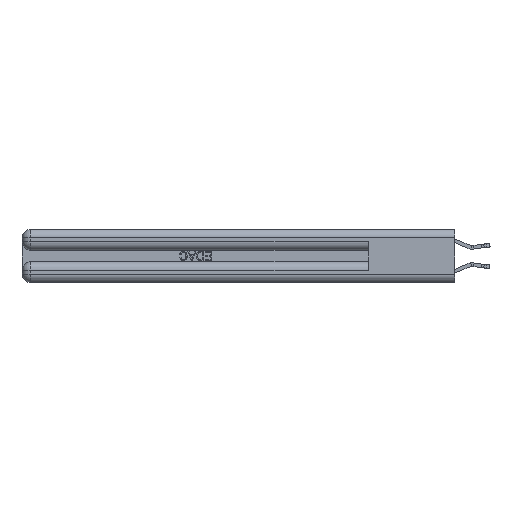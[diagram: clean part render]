
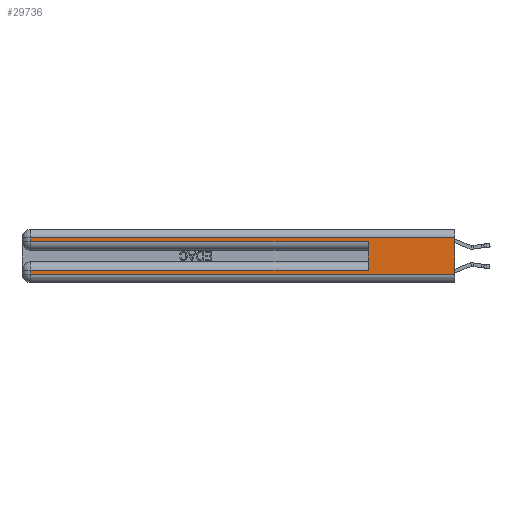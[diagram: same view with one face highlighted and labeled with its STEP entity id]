
A CAD part, left-side view. The second image highlights one B-rep face of the part: STEP entity #29736.
In plain terms, the highlighted planar face has unit normal (-1, 0, 0).
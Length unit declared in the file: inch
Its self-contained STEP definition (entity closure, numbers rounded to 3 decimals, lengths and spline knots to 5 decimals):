
#534 = VERTEX_POINT ( 'NONE', #14235 ) ;
#927 = EDGE_CURVE ( 'NONE', #534, #16328, #31552, .T. ) ;
#960 = VECTOR ( 'NONE', #29617, 39.37008 ) ;
#1057 = ORIENTED_EDGE ( 'NONE', *, *, #927, .F. ) ;
#1247 = DIRECTION ( 'NONE',  ( 0., 0., -1. ) ) ;
#2340 = LINE ( 'NONE', #7037, #28582 ) ;
#2601 = ORIENTED_EDGE ( 'NONE', *, *, #12074, .F. ) ;
#3421 = CARTESIAN_POINT ( 'NONE',  ( 0., 2.94, 0.37 ) ) ;
#4107 = ORIENTED_EDGE ( 'NONE', *, *, #19703, .T. ) ;
#4327 = DIRECTION ( 'NONE',  ( 0., 0., -1. ) ) ;
#4560 = CARTESIAN_POINT ( 'NONE',  ( 0., 2.94, 0.31 ) ) ;
#4582 = EDGE_CURVE ( 'NONE', #31586, #15695, #20592, .T. ) ;
#4812 = LINE ( 'NONE', #3421, #18489 ) ;
#4942 = CARTESIAN_POINT ( 'NONE',  ( 0., 0., 0.285 ) ) ;
#4948 = CARTESIAN_POINT ( 'NONE',  ( 0., 2.94, 0.285 ) ) ;
#5281 = EDGE_CURVE ( 'NONE', #27657, #31586, #29476, .T. ) ;
#5358 = VERTEX_POINT ( 'NONE', #4948 ) ;
#6034 = VECTOR ( 'NONE', #18473, 39.37008 ) ;
#6879 = VECTOR ( 'NONE', #26923, 39.37008 ) ;
#7037 = CARTESIAN_POINT ( 'NONE',  ( 0., 0.6, 0.145 ) ) ;
#8656 = AXIS2_PLACEMENT_3D ( 'NONE', #24034, #32707, #4327 ) ;
#8777 = VECTOR ( 'NONE', #22987, 39.37008 ) ;
#8871 = CARTESIAN_POINT ( 'NONE',  ( 0., 2.94, 0.085 ) ) ;
#9125 = EDGE_LOOP ( 'NONE', ( #1057, #27682, #4107, #14653, #2601, #18372, #16682, #28403 ) ) ;
#9712 = DIRECTION ( 'NONE',  ( 0., 0., 1. ) ) ;
#10415 = FACE_OUTER_BOUND ( 'NONE', #9125, .T. ) ;
#12026 = VERTEX_POINT ( 'NONE', #4560 ) ;
#12074 = EDGE_CURVE ( 'NONE', #27657, #14580, #2340, .T. ) ;
#12557 = CARTESIAN_POINT ( 'NONE',  ( 0., 2.94, 0.06 ) ) ;
#12581 = CARTESIAN_POINT ( 'NONE',  ( 0., 0., 0.31 ) ) ;
#13320 = CARTESIAN_POINT ( 'NONE',  ( 0., 0.6, 0.085 ) ) ;
#14235 = CARTESIAN_POINT ( 'NONE',  ( 0., 0., 0.31 ) ) ;
#14580 = VERTEX_POINT ( 'NONE', #17454 ) ;
#14653 = ORIENTED_EDGE ( 'NONE', *, *, #20606, .T. ) ;
#15695 = VERTEX_POINT ( 'NONE', #12557 ) ;
#16206 = CARTESIAN_POINT ( 'NONE',  ( 0., 0., 0.06 ) ) ;
#16328 = VERTEX_POINT ( 'NONE', #29044 ) ;
#16490 = EDGE_CURVE ( 'NONE', #15695, #16328, #23531, .T. ) ;
#16682 = ORIENTED_EDGE ( 'NONE', *, *, #4582, .T. ) ;
#17454 = CARTESIAN_POINT ( 'NONE',  ( 0., 0.6, 0.285 ) ) ;
#18372 = ORIENTED_EDGE ( 'NONE', *, *, #5281, .T. ) ;
#18473 = DIRECTION ( 'NONE',  ( 0., 1., 0. ) ) ;
#18489 = VECTOR ( 'NONE', #23803, 39.37008 ) ;
#19703 = EDGE_CURVE ( 'NONE', #12026, #5358, #4812, .T. ) ;
#20592 = LINE ( 'NONE', #32036, #6879 ) ;
#20606 = EDGE_CURVE ( 'NONE', #5358, #14580, #24117, .T. ) ;
#22987 = DIRECTION ( 'NONE',  ( 0., -1., 0. ) ) ;
#23531 = LINE ( 'NONE', #16206, #960 ) ;
#23803 = DIRECTION ( 'NONE',  ( 0., 0., -1. ) ) ;
#24034 = CARTESIAN_POINT ( 'NONE',  ( 0., 0., 0.37 ) ) ;
#24117 = LINE ( 'NONE', #4942, #8777 ) ;
#24937 = PLANE ( 'NONE',  #8656 ) ;
#25342 = DIRECTION ( 'NONE',  ( 0., 1., 0. ) ) ;
#26923 = DIRECTION ( 'NONE',  ( 0., 0., -1. ) ) ;
#27657 = VERTEX_POINT ( 'NONE', #13320 ) ;
#27682 = ORIENTED_EDGE ( 'NONE', *, *, #31953, .T. ) ;
#28337 = CARTESIAN_POINT ( 'NONE',  ( 0., 0., 0.085 ) ) ;
#28403 = ORIENTED_EDGE ( 'NONE', *, *, #16490, .T. ) ;
#28582 = VECTOR ( 'NONE', #9712, 39.37008 ) ;
#28873 = VECTOR ( 'NONE', #25342, 39.37008 ) ;
#29044 = CARTESIAN_POINT ( 'NONE',  ( 0., 0., 0.06 ) ) ;
#29476 = LINE ( 'NONE', #28337, #6034 ) ;
#29617 = DIRECTION ( 'NONE',  ( 0., -1., 0. ) ) ;
#29736 = ADVANCED_FACE ( 'NONE', ( #10415 ), #24937, .F. ) ;
#30737 = VECTOR ( 'NONE', #1247, 39.37008 ) ;
#31552 = LINE ( 'NONE', #32325, #30737 ) ;
#31586 = VERTEX_POINT ( 'NONE', #8871 ) ;
#31731 = LINE ( 'NONE', #12581, #28873 ) ;
#31953 = EDGE_CURVE ( 'NONE', #534, #12026, #31731, .T. ) ;
#32036 = CARTESIAN_POINT ( 'NONE',  ( 0., 2.94, 0.37 ) ) ;
#32325 = CARTESIAN_POINT ( 'NONE',  ( 0., 0., 0.37 ) ) ;
#32707 = DIRECTION ( 'NONE',  ( 1., 0., 0. ) ) ;
